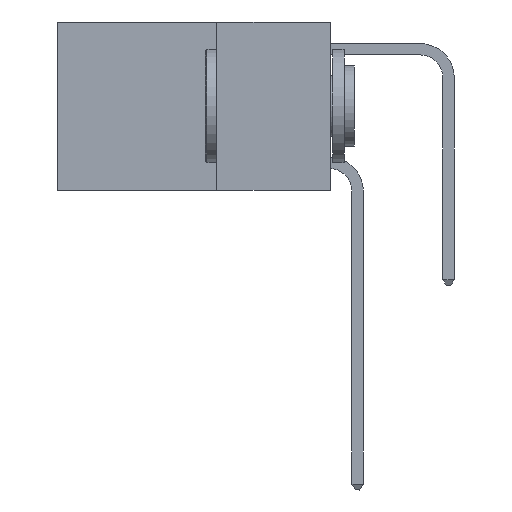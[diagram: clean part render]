
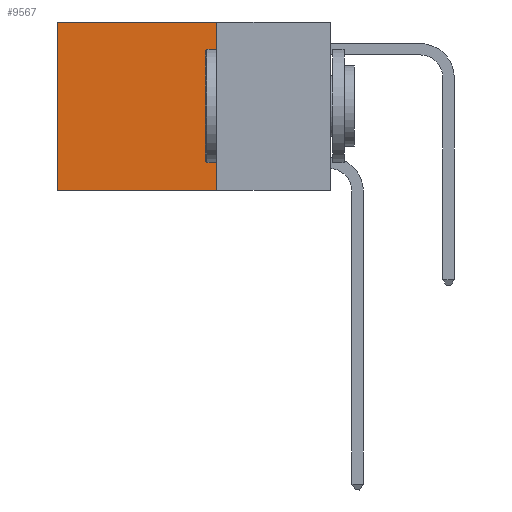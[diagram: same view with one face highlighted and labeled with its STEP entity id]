
A CAD part, left-side view. The second image highlights one B-rep face of the part: STEP entity #9567.
In plain terms, the highlighted planar face has unit normal (-1, 0, 0).
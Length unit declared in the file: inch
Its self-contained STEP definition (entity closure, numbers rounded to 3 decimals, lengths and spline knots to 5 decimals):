
#334 = LINE ( 'NONE', #1871, #20645 ) ;
#632 = CARTESIAN_POINT ( 'NONE',  ( 0.2625, 0.25, 0. ) ) ;
#676 = CARTESIAN_POINT ( 'NONE',  ( 0.2625, 0.25, 0. ) ) ;
#814 = ORIENTED_EDGE ( 'NONE', *, *, #3572, .F. ) ;
#1814 = VECTOR ( 'NONE', #18659, 39.37008 ) ;
#1871 = CARTESIAN_POINT ( 'NONE',  ( 0.2625, 0.6, 0. ) ) ;
#2442 = VECTOR ( 'NONE', #13600, 39.37008 ) ;
#3572 = EDGE_CURVE ( 'NONE', #20451, #19439, #4835, .T. ) ;
#4065 = FACE_OUTER_BOUND ( 'NONE', #8350, .T. ) ;
#4481 = CARTESIAN_POINT ( 'NONE',  ( 0.2625, 0.25, 0. ) ) ;
#4835 = LINE ( 'NONE', #20706, #1814 ) ;
#5183 = VECTOR ( 'NONE', #20092, 39.37008 ) ;
#7378 = EDGE_CURVE ( 'NONE', #21421, #16755, #7622, .T. ) ;
#7622 = LINE ( 'NONE', #23023, #2442 ) ;
#7869 = CARTESIAN_POINT ( 'NONE',  ( 0.2625, 0.6, 0. ) ) ;
#8079 = DIRECTION ( 'NONE',  ( 0., 0., -1. ) ) ;
#8112 = DIRECTION ( 'NONE',  ( 1., 0., 0. ) ) ;
#8350 = EDGE_LOOP ( 'NONE', ( #13949, #814, #23587, #19245 ) ) ;
#8641 = EDGE_CURVE ( 'NONE', #16755, #19439, #334, .T. ) ;
#9567 = ADVANCED_FACE ( 'NONE', ( #4065 ), #21855, .F. ) ;
#10991 = EDGE_CURVE ( 'NONE', #21421, #20451, #20344, .T. ) ;
#13600 = DIRECTION ( 'NONE',  ( 0., 1., 0. ) ) ;
#13949 = ORIENTED_EDGE ( 'NONE', *, *, #8641, .T. ) ;
#15503 = CARTESIAN_POINT ( 'NONE',  ( 0.2625, 0.25, -0.37 ) ) ;
#16755 = VERTEX_POINT ( 'NONE', #7869 ) ;
#17819 = AXIS2_PLACEMENT_3D ( 'NONE', #632, #8112, #23510 ) ;
#18659 = DIRECTION ( 'NONE',  ( 0., 1., 0. ) ) ;
#19245 = ORIENTED_EDGE ( 'NONE', *, *, #7378, .T. ) ;
#19439 = VERTEX_POINT ( 'NONE', #21990 ) ;
#20092 = DIRECTION ( 'NONE',  ( 0., 0., -1. ) ) ;
#20344 = LINE ( 'NONE', #4481, #5183 ) ;
#20451 = VERTEX_POINT ( 'NONE', #15503 ) ;
#20645 = VECTOR ( 'NONE', #8079, 39.37008 ) ;
#20706 = CARTESIAN_POINT ( 'NONE',  ( 0.2625, 0.25, -0.37 ) ) ;
#21421 = VERTEX_POINT ( 'NONE', #676 ) ;
#21855 = PLANE ( 'NONE',  #17819 ) ;
#21990 = CARTESIAN_POINT ( 'NONE',  ( 0.2625, 0.6, -0.37 ) ) ;
#23023 = CARTESIAN_POINT ( 'NONE',  ( 0.2625, 0.25, 0. ) ) ;
#23510 = DIRECTION ( 'NONE',  ( 0., 0., -1. ) ) ;
#23587 = ORIENTED_EDGE ( 'NONE', *, *, #10991, .F. ) ;
